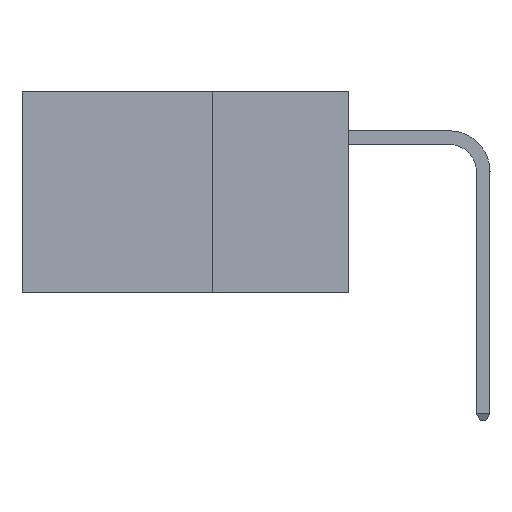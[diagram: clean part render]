
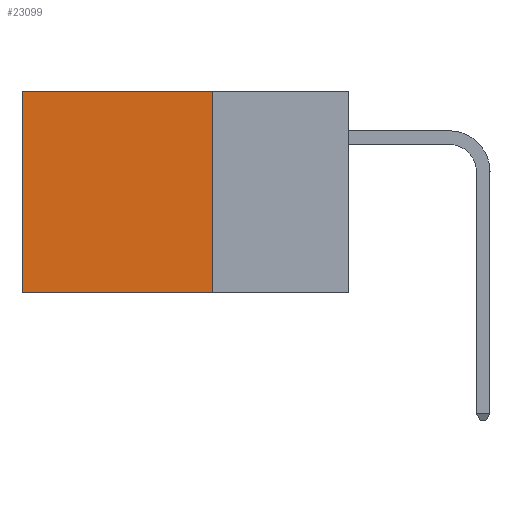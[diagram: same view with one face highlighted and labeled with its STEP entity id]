
A CAD part, left-side view. The second image highlights one B-rep face of the part: STEP entity #23099.
In plain terms, the highlighted planar face has unit normal (-1, 0, 0).
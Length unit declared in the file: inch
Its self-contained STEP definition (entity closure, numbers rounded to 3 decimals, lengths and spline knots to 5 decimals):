
#719 = ORIENTED_EDGE ( 'NONE', *, *, #22999, .T. ) ;
#1449 = DIRECTION ( 'NONE',  ( 0., 1., 0. ) ) ;
#1872 = CARTESIAN_POINT ( 'NONE',  ( 0.2875, 0.6, -0.37 ) ) ;
#3139 = CARTESIAN_POINT ( 'NONE',  ( 0.2875, 0.25, 0. ) ) ;
#3292 = LINE ( 'NONE', #12916, #23208 ) ;
#3499 = PLANE ( 'NONE',  #26067 ) ;
#3648 = VERTEX_POINT ( 'NONE', #35815 ) ;
#3759 = VECTOR ( 'NONE', #11809, 39.37008 ) ;
#4702 = EDGE_CURVE ( 'NONE', #15262, #29539, #3292, .T. ) ;
#5238 = DIRECTION ( 'NONE',  ( 0., 0., -1. ) ) ;
#5874 = LINE ( 'NONE', #13572, #12604 ) ;
#6283 = EDGE_CURVE ( 'NONE', #3648, #29539, #5874, .T. ) ;
#7309 = CARTESIAN_POINT ( 'NONE',  ( 0.2875, 0.25, 0. ) ) ;
#7831 = CARTESIAN_POINT ( 'NONE',  ( 0.2875, 0.25, -0.37 ) ) ;
#9293 = VERTEX_POINT ( 'NONE', #7309 ) ;
#9310 = CARTESIAN_POINT ( 'NONE',  ( 0.2875, 0.25, 0. ) ) ;
#11019 = CARTESIAN_POINT ( 'NONE',  ( 0.2875, 0.25, 0. ) ) ;
#11421 = LINE ( 'NONE', #3139, #3759 ) ;
#11809 = DIRECTION ( 'NONE',  ( 0., 1., 0. ) ) ;
#11976 = EDGE_CURVE ( 'NONE', #9293, #15262, #12219, .T. ) ;
#12173 = DIRECTION ( 'NONE',  ( 1., 0., 0. ) ) ;
#12219 = LINE ( 'NONE', #11019, #33465 ) ;
#12604 = VECTOR ( 'NONE', #19089, 39.37008 ) ;
#12916 = CARTESIAN_POINT ( 'NONE',  ( 0.2875, 0.25, -0.37 ) ) ;
#13572 = CARTESIAN_POINT ( 'NONE',  ( 0.2875, 0.6, 0. ) ) ;
#14490 = ORIENTED_EDGE ( 'NONE', *, *, #11976, .F. ) ;
#15262 = VERTEX_POINT ( 'NONE', #7831 ) ;
#15414 = EDGE_LOOP ( 'NONE', ( #21919, #36009, #14490, #719 ) ) ;
#19089 = DIRECTION ( 'NONE',  ( 0., 0., -1. ) ) ;
#21919 = ORIENTED_EDGE ( 'NONE', *, *, #6283, .T. ) ;
#22999 = EDGE_CURVE ( 'NONE', #9293, #3648, #11421, .T. ) ;
#23099 = ADVANCED_FACE ( 'NONE', ( #30969 ), #3499, .F. ) ;
#23208 = VECTOR ( 'NONE', #1449, 39.37008 ) ;
#26067 = AXIS2_PLACEMENT_3D ( 'NONE', #9310, #12173, #31556 ) ;
#29539 = VERTEX_POINT ( 'NONE', #1872 ) ;
#30969 = FACE_OUTER_BOUND ( 'NONE', #15414, .T. ) ;
#31556 = DIRECTION ( 'NONE',  ( 0., 0., -1. ) ) ;
#33465 = VECTOR ( 'NONE', #5238, 39.37008 ) ;
#35815 = CARTESIAN_POINT ( 'NONE',  ( 0.2875, 0.6, 0. ) ) ;
#36009 = ORIENTED_EDGE ( 'NONE', *, *, #4702, .F. ) ;
